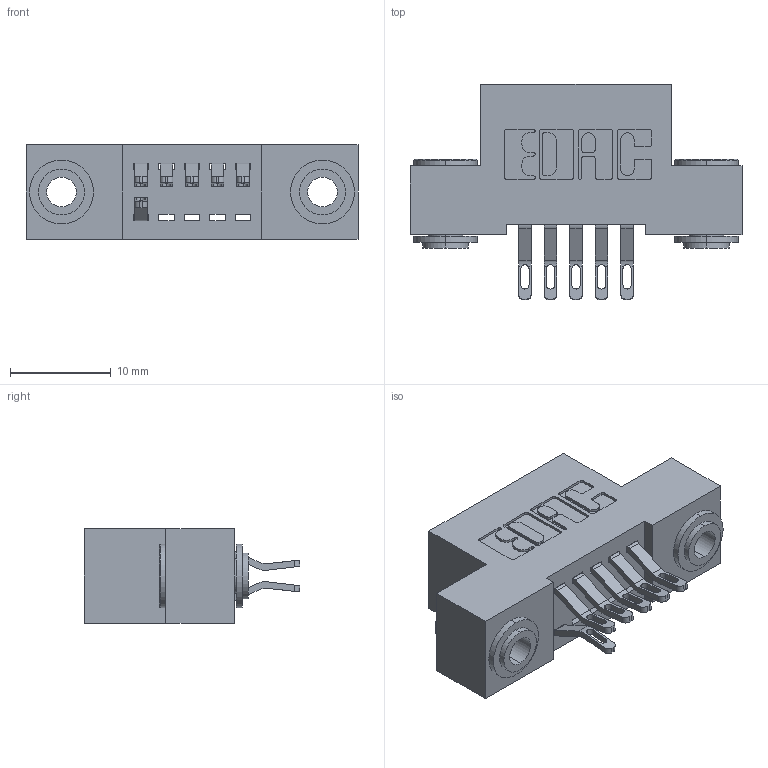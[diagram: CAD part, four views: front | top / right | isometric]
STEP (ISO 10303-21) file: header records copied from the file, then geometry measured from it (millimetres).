
FILE_DESCRIPTION (( 'STEP AP203' ), '1' );
FILE_NAME ('392-010-555-203.STEP', '2018-08-14T20:47:57', ( '' ), ( '' ), 'SwSTEP 2.0', 'SolidWorks 2016', '' );
FILE_SCHEMA (( 'CONFIG_CONTROL_DESIGN' ));
Length unit declared in the file: inch
Products named in the file (4): 342 Part_.156 TH; 345-292-001_555 Tail; 342-250-002_345-250-002-102; 392-010-555-203
Assembly tree (9 placements, depth 2):
  392-010-555-203
    342 Part_.156 TH
    345-292-001_555 Tail  x6
    342-250-002_345-250-002-102  x2
Bounding box: 33.02 x 21.47 x 9.4 mm (x, y, z)
Volume: 2795.2 mm3; surface area: 3711.4 mm2
Topology: 9 solids, 9 shells, 520 faces, 1557 edges, 1034 vertices
Faces by surface type: plane 304, cylinder 208, cone 8
Entity records: 8718 total; most frequent: CARTESIAN_POINT 1515, ORIENTED_EDGE 1418, DIRECTION 1359, EDGE_CURVE 709, VECTOR 537, LINE 537, VERTEX_POINT 470, AXIS2_PLACEMENT_3D 411
